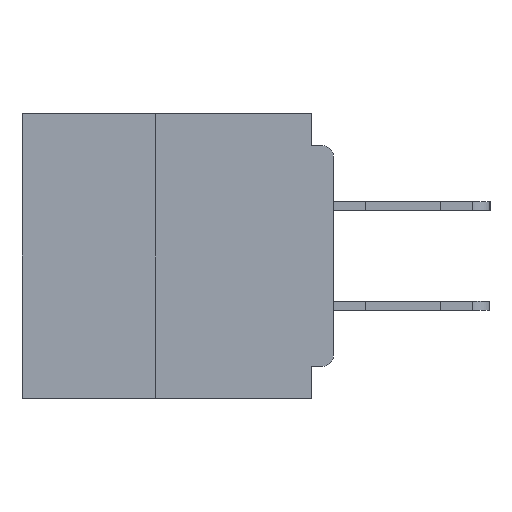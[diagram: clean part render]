
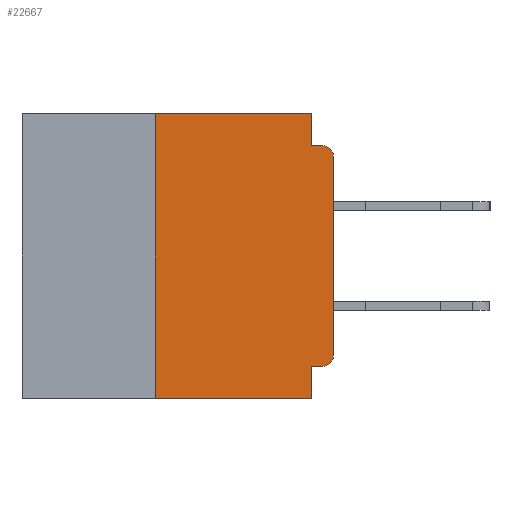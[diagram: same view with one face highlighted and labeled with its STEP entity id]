
A CAD part, left-side view. The second image highlights one B-rep face of the part: STEP entity #22667.
In plain terms, the highlighted planar face has unit normal (-1, 0, 0).
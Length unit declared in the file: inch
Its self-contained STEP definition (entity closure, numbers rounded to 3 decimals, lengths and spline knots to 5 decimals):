
#790 = LINE ( 'NONE', #50759, #46607 ) ;
#1660 = DIRECTION ( 'NONE',  ( -1., 0., 0. ) ) ;
#2672 = VERTEX_POINT ( 'NONE', #4185 ) ;
#3329 = ORIENTED_EDGE ( 'NONE', *, *, #4091, .T. ) ;
#4091 = EDGE_CURVE ( 'NONE', #12614, #32295, #32895, .T. ) ;
#4185 = CARTESIAN_POINT ( 'NONE',  ( 0., 0.031, -0.045 ) ) ;
#4457 = DIRECTION ( 'NONE',  ( 0., 0., 1. ) ) ;
#4509 = ORIENTED_EDGE ( 'NONE', *, *, #7070, .F. ) ;
#7070 = EDGE_CURVE ( 'NONE', #12614, #12472, #46531, .T. ) ;
#7521 = CARTESIAN_POINT ( 'NONE',  ( 0., 0.25, 0. ) ) ;
#8877 = AXIS2_PLACEMENT_3D ( 'NONE', #49323, #22730, #53791 ) ;
#9131 = CARTESIAN_POINT ( 'NONE',  ( 0., 0., -0.355 ) ) ;
#9336 = VERTEX_POINT ( 'NONE', #26534 ) ;
#9363 = EDGE_CURVE ( 'NONE', #17275, #48897, #10241, .T. ) ;
#9791 = VECTOR ( 'NONE', #40124, 39.37008 ) ;
#10037 = EDGE_CURVE ( 'NONE', #9336, #2672, #56599, .T. ) ;
#10241 = LINE ( 'NONE', #44391, #44242 ) ;
#10920 = DIRECTION ( 'NONE',  ( 0., 0., -1. ) ) ;
#11128 = VECTOR ( 'NONE', #26464, 39.37008 ) ;
#12472 = VERTEX_POINT ( 'NONE', #7521 ) ;
#12614 = VERTEX_POINT ( 'NONE', #26292 ) ;
#14094 = DIRECTION ( 'NONE',  ( 0., -1., 0. ) ) ;
#17275 = VERTEX_POINT ( 'NONE', #19087 ) ;
#17899 = CARTESIAN_POINT ( 'NONE',  ( 0., 0., -0.045 ) ) ;
#19087 = CARTESIAN_POINT ( 'NONE',  ( 0., 0., -0.34 ) ) ;
#21056 = VECTOR ( 'NONE', #14094, 39.37008 ) ;
#21450 = AXIS2_PLACEMENT_3D ( 'NONE', #28202, #1660, #32697 ) ;
#21561 = LINE ( 'NONE', #9131, #9791 ) ;
#22006 = CARTESIAN_POINT ( 'NONE',  ( 0., 0.25, -0.4 ) ) ;
#22403 = CARTESIAN_POINT ( 'NONE',  ( 0., 0.031, 0. ) ) ;
#22667 = ADVANCED_FACE ( 'NONE', ( #50966 ), #41583, .F. ) ;
#22730 = DIRECTION ( 'NONE',  ( -1., 0., 0. ) ) ;
#23966 = CARTESIAN_POINT ( 'NONE',  ( 0., 0.437, 0. ) ) ;
#26200 = AXIS2_PLACEMENT_3D ( 'NONE', #23966, #54999, #28438 ) ;
#26292 = CARTESIAN_POINT ( 'NONE',  ( 0., 0.25, -0.4 ) ) ;
#26414 = EDGE_CURVE ( 'NONE', #37487, #17275, #47385, .T. ) ;
#26464 = DIRECTION ( 'NONE',  ( 0., 0., 1. ) ) ;
#26534 = CARTESIAN_POINT ( 'NONE',  ( 0., 0.031, 0. ) ) ;
#27841 = CARTESIAN_POINT ( 'NONE',  ( 0., 0.015, -0.045 ) ) ;
#28202 = CARTESIAN_POINT ( 'NONE',  ( 0., 0.015, -0.06 ) ) ;
#28438 = DIRECTION ( 'NONE',  ( 0., 0., -1. ) ) ;
#32295 = VERTEX_POINT ( 'NONE', #34817 ) ;
#32697 = DIRECTION ( 'NONE',  ( 0., 0., -1. ) ) ;
#32895 = LINE ( 'NONE', #40635, #21056 ) ;
#34276 = EDGE_CURVE ( 'NONE', #2672, #48005, #50452, .T. ) ;
#34775 = CARTESIAN_POINT ( 'NONE',  ( 0., 0., -0.06 ) ) ;
#34817 = CARTESIAN_POINT ( 'NONE',  ( 0., 0.031, -0.4 ) ) ;
#34904 = ORIENTED_EDGE ( 'NONE', *, *, #49813, .F. ) ;
#35207 = CARTESIAN_POINT ( 'NONE',  ( 0., 0.031, -0.355 ) ) ;
#35783 = DIRECTION ( 'NONE',  ( 0., -1., 0. ) ) ;
#36181 = ORIENTED_EDGE ( 'NONE', *, *, #41842, .F. ) ;
#37244 = VECTOR ( 'NONE', #35783, 39.37008 ) ;
#37487 = VERTEX_POINT ( 'NONE', #54724 ) ;
#38118 = ORIENTED_EDGE ( 'NONE', *, *, #9363, .T. ) ;
#38306 = CIRCLE ( 'NONE', #21450, 0.015 ) ;
#38995 = VERTEX_POINT ( 'NONE', #35207 ) ;
#39661 = ORIENTED_EDGE ( 'NONE', *, *, #34276, .F. ) ;
#40124 = DIRECTION ( 'NONE',  ( 0., 1., 0. ) ) ;
#40635 = CARTESIAN_POINT ( 'NONE',  ( 0., 0.437, -0.4 ) ) ;
#41583 = PLANE ( 'NONE',  #26200 ) ;
#41842 = EDGE_CURVE ( 'NONE', #12472, #9336, #790, .T. ) ;
#41916 = CARTESIAN_POINT ( 'NONE',  ( 0., 0.031, -0.4 ) ) ;
#41971 = ORIENTED_EDGE ( 'NONE', *, *, #50252, .F. ) ;
#43827 = VECTOR ( 'NONE', #10920, 39.37008 ) ;
#44242 = VECTOR ( 'NONE', #4457, 39.37008 ) ;
#44258 = EDGE_CURVE ( 'NONE', #48897, #48005, #38306, .T. ) ;
#44391 = CARTESIAN_POINT ( 'NONE',  ( 0., 0., 0. ) ) ;
#44449 = ORIENTED_EDGE ( 'NONE', *, *, #26414, .T. ) ;
#44535 = DIRECTION ( 'NONE',  ( 0., 0., -1. ) ) ;
#44678 = ORIENTED_EDGE ( 'NONE', *, *, #44258, .T. ) ;
#46531 = LINE ( 'NONE', #22006, #11128 ) ;
#46607 = VECTOR ( 'NONE', #55181, 39.37008 ) ;
#47385 = CIRCLE ( 'NONE', #8877, 0.015 ) ;
#48005 = VERTEX_POINT ( 'NONE', #27841 ) ;
#48897 = VERTEX_POINT ( 'NONE', #34775 ) ;
#49323 = CARTESIAN_POINT ( 'NONE',  ( 0., 0.015, -0.34 ) ) ;
#49615 = EDGE_LOOP ( 'NONE', ( #38118, #44678, #39661, #50764, #36181, #4509, #3329, #34904, #41971, #44449 ) ) ;
#49813 = EDGE_CURVE ( 'NONE', #38995, #32295, #55611, .T. ) ;
#50252 = EDGE_CURVE ( 'NONE', #37487, #38995, #21561, .T. ) ;
#50452 = LINE ( 'NONE', #17899, #37244 ) ;
#50759 = CARTESIAN_POINT ( 'NONE',  ( 0., 0.437, 0. ) ) ;
#50764 = ORIENTED_EDGE ( 'NONE', *, *, #10037, .F. ) ;
#50966 = FACE_OUTER_BOUND ( 'NONE', #49615, .T. ) ;
#53791 = DIRECTION ( 'NONE',  ( 0., 0., -1. ) ) ;
#54724 = CARTESIAN_POINT ( 'NONE',  ( 0., 0.015, -0.355 ) ) ;
#54999 = DIRECTION ( 'NONE',  ( 1., 0., 0. ) ) ;
#55181 = DIRECTION ( 'NONE',  ( 0., -1., 0. ) ) ;
#55250 = VECTOR ( 'NONE', #44535, 39.37008 ) ;
#55611 = LINE ( 'NONE', #41916, #43827 ) ;
#56599 = LINE ( 'NONE', #22403, #55250 ) ;
